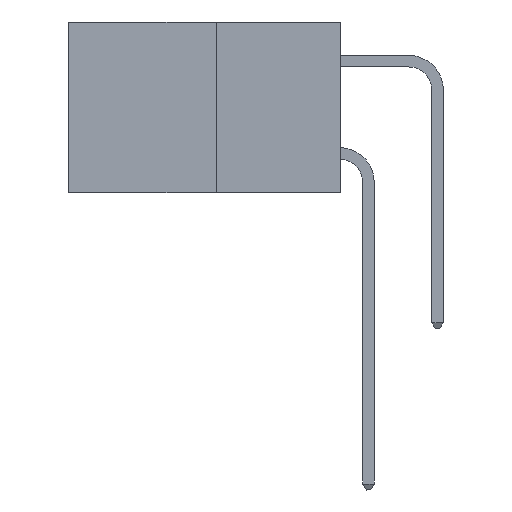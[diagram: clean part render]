
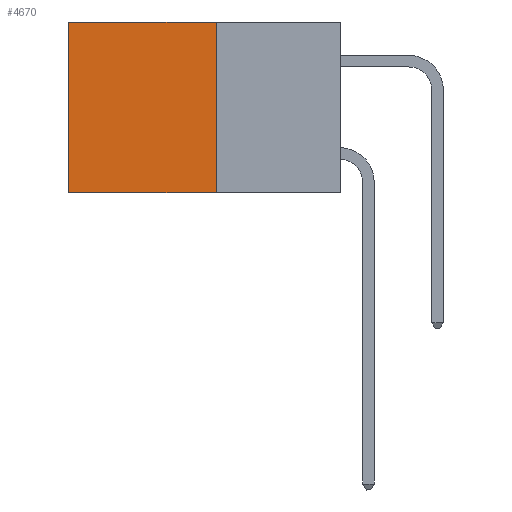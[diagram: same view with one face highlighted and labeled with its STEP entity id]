
A CAD part, left-side view. The second image highlights one B-rep face of the part: STEP entity #4670.
In plain terms, the highlighted planar face has unit normal (-1, 0, 0).
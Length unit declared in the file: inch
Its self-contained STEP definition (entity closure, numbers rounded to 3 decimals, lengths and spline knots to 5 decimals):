
#196 = EDGE_CURVE ( 'NONE', #9467, #2895, #2210, .T. ) ;
#696 = DIRECTION ( 'NONE',  ( 1., 0., 0. ) ) ;
#1448 = CARTESIAN_POINT ( 'NONE',  ( 0.277, 0.27, -0.37 ) ) ;
#2117 = VECTOR ( 'NONE', #11224, 39.37008 ) ;
#2210 = LINE ( 'NONE', #1448, #9146 ) ;
#2890 = VERTEX_POINT ( 'NONE', #7188 ) ;
#2895 = VERTEX_POINT ( 'NONE', #7154 ) ;
#3687 = CARTESIAN_POINT ( 'NONE',  ( 0.277, 0.59, -0.37 ) ) ;
#3967 = ORIENTED_EDGE ( 'NONE', *, *, #5171, .F. ) ;
#4199 = CARTESIAN_POINT ( 'NONE',  ( 0.277, 0.27, 0. ) ) ;
#4296 = VECTOR ( 'NONE', #11356, 39.37008 ) ;
#4670 = ADVANCED_FACE ( 'NONE', ( #7087 ), #11991, .F. ) ;
#5171 = EDGE_CURVE ( 'NONE', #2895, #6529, #12499, .T. ) ;
#5863 = CARTESIAN_POINT ( 'NONE',  ( 0.277, 0.27, -0.37 ) ) ;
#6035 = DIRECTION ( 'NONE',  ( 0., 0., -1. ) ) ;
#6076 = EDGE_CURVE ( 'NONE', #9467, #2890, #11161, .T. ) ;
#6529 = VERTEX_POINT ( 'NONE', #3687 ) ;
#7087 = FACE_OUTER_BOUND ( 'NONE', #12764, .T. ) ;
#7154 = CARTESIAN_POINT ( 'NONE',  ( 0.277, 0.27, -0.37 ) ) ;
#7188 = CARTESIAN_POINT ( 'NONE',  ( 0.277, 0.59, 0. ) ) ;
#7492 = CARTESIAN_POINT ( 'NONE',  ( 0.277, 0.59, -0.37 ) ) ;
#8158 = DIRECTION ( 'NONE',  ( 0., 0., -1. ) ) ;
#8738 = ORIENTED_EDGE ( 'NONE', *, *, #8813, .T. ) ;
#8813 = EDGE_CURVE ( 'NONE', #2890, #6529, #11613, .T. ) ;
#9146 = VECTOR ( 'NONE', #6035, 39.37008 ) ;
#9467 = VERTEX_POINT ( 'NONE', #4199 ) ;
#9684 = VECTOR ( 'NONE', #12674, 39.37008 ) ;
#10256 = CARTESIAN_POINT ( 'NONE',  ( 0.277, 0.27, 0. ) ) ;
#10421 = AXIS2_PLACEMENT_3D ( 'NONE', #12925, #696, #8158 ) ;
#11161 = LINE ( 'NONE', #10256, #2117 ) ;
#11166 = ORIENTED_EDGE ( 'NONE', *, *, #6076, .T. ) ;
#11224 = DIRECTION ( 'NONE',  ( 0., 1., 0. ) ) ;
#11356 = DIRECTION ( 'NONE',  ( 0., 0., -1. ) ) ;
#11613 = LINE ( 'NONE', #7492, #4296 ) ;
#11905 = ORIENTED_EDGE ( 'NONE', *, *, #196, .F. ) ;
#11991 = PLANE ( 'NONE',  #10421 ) ;
#12499 = LINE ( 'NONE', #5863, #9684 ) ;
#12674 = DIRECTION ( 'NONE',  ( 0., 1., 0. ) ) ;
#12764 = EDGE_LOOP ( 'NONE', ( #8738, #3967, #11905, #11166 ) ) ;
#12925 = CARTESIAN_POINT ( 'NONE',  ( 0.277, 0.27, -0.37 ) ) ;
